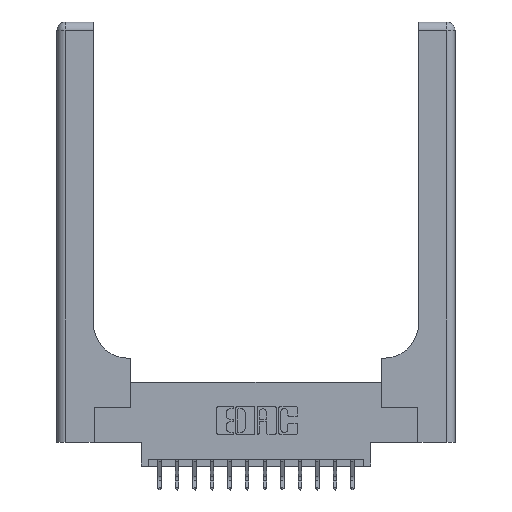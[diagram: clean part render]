
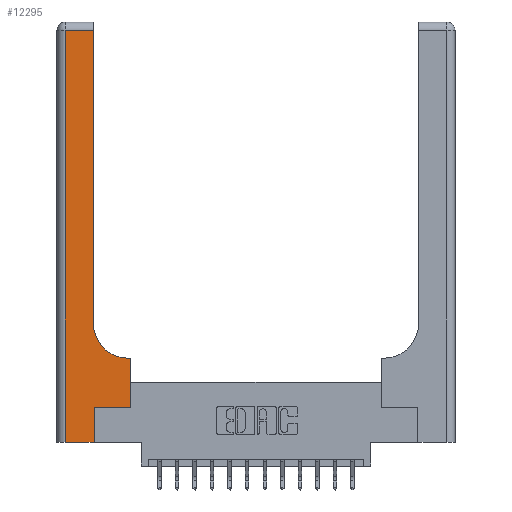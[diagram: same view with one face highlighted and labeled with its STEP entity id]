
A CAD part, top view. The second image highlights one B-rep face of the part: STEP entity #12295.
In plain terms, the highlighted planar face has unit normal (0, 0, 1).
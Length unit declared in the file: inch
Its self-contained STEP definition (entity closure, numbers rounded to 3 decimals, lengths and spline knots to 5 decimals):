
#17 = VECTOR ( 'NONE', #10789, 39.37008 ) ;
#334 = LINE ( 'NONE', #4444, #10123 ) ;
#576 = LINE ( 'NONE', #14651, #10993 ) ;
#1118 = VERTEX_POINT ( 'NONE', #5694 ) ;
#1309 = AXIS2_PLACEMENT_3D ( 'NONE', #10838, #9506, #16489 ) ;
#1325 = VERTEX_POINT ( 'NONE', #16546 ) ;
#1569 = ORIENTED_EDGE ( 'NONE', *, *, #14735, .T. ) ;
#2502 = VERTEX_POINT ( 'NONE', #8086 ) ;
#2768 = EDGE_CURVE ( 'NONE', #1325, #4122, #14981, .T. ) ;
#3259 = DIRECTION ( 'NONE',  ( 0., -1., 0. ) ) ;
#3391 = LINE ( 'NONE', #16825, #10990 ) ;
#3487 = AXIS2_PLACEMENT_3D ( 'NONE', #13956, #15382, #6989 ) ;
#3611 = CARTESIAN_POINT ( 'NONE',  ( 0.06, 0., 0.37 ) ) ;
#3619 = LINE ( 'NONE', #14592, #6126 ) ;
#3621 = ORIENTED_EDGE ( 'NONE', *, *, #2768, .T. ) ;
#4122 = VERTEX_POINT ( 'NONE', #6621 ) ;
#4444 = CARTESIAN_POINT ( 'NONE',  ( 0.06, 3., 0.37 ) ) ;
#4776 = ORIENTED_EDGE ( 'NONE', *, *, #13114, .T. ) ;
#4876 = EDGE_CURVE ( 'NONE', #17245, #13793, #6513, .T. ) ;
#4936 = EDGE_CURVE ( 'NONE', #9885, #12798, #14653, .T. ) ;
#5588 = CARTESIAN_POINT ( 'NONE',  ( 0.528, 0.25, 0.37 ) ) ;
#5694 = CARTESIAN_POINT ( 'NONE',  ( 0.06, 2.94, 0.37 ) ) ;
#5962 = DIRECTION ( 'NONE',  ( 1., 0., 0. ) ) ;
#6100 = VECTOR ( 'NONE', #9036, 39.37008 ) ;
#6126 = VECTOR ( 'NONE', #8880, 39.37008 ) ;
#6250 = DIRECTION ( 'NONE',  ( -1., 0., 0. ) ) ;
#6513 = LINE ( 'NONE', #10456, #6100 ) ;
#6621 = CARTESIAN_POINT ( 'NONE',  ( 0.26, 2.94, 0.37 ) ) ;
#6989 = DIRECTION ( 'NONE',  ( -1., 0., 0. ) ) ;
#7550 = VECTOR ( 'NONE', #14741, 39.37008 ) ;
#7786 = EDGE_CURVE ( 'NONE', #2502, #17245, #3391, .T. ) ;
#8086 = CARTESIAN_POINT ( 'NONE',  ( 0.265, 0.25, 0.37 ) ) ;
#8865 = CIRCLE ( 'NONE', #1309, 0.25 ) ;
#8880 = DIRECTION ( 'NONE',  ( -1., 0., 0. ) ) ;
#9036 = DIRECTION ( 'NONE',  ( 0., 1., 0. ) ) ;
#9077 = CARTESIAN_POINT ( 'NONE',  ( 0.265, 0., 0.37 ) ) ;
#9306 = CARTESIAN_POINT ( 'NONE',  ( 0., 0., 0.37 ) ) ;
#9506 = DIRECTION ( 'NONE',  ( 0., 0., -1. ) ) ;
#9885 = VERTEX_POINT ( 'NONE', #3611 ) ;
#10052 = EDGE_CURVE ( 'NONE', #14699, #1325, #8865, .T. ) ;
#10123 = VECTOR ( 'NONE', #3259, 39.37008 ) ;
#10176 = ORIENTED_EDGE ( 'NONE', *, *, #4876, .T. ) ;
#10443 = ORIENTED_EDGE ( 'NONE', *, *, #16587, .T. ) ;
#10456 = CARTESIAN_POINT ( 'NONE',  ( 0.528, 0.25, 0.37 ) ) ;
#10625 = CARTESIAN_POINT ( 'NONE',  ( 0.51, 0.6, 0.37 ) ) ;
#10789 = DIRECTION ( 'NONE',  ( 0., 1., 0. ) ) ;
#10838 = CARTESIAN_POINT ( 'NONE',  ( 0.51, 0.85, 0.37 ) ) ;
#10990 = VECTOR ( 'NONE', #5962, 39.37008 ) ;
#10993 = VECTOR ( 'NONE', #14485, 39.37008 ) ;
#12072 = CARTESIAN_POINT ( 'NONE',  ( 0.528, 0.6, 0.37 ) ) ;
#12295 = ADVANCED_FACE ( 'NONE', ( #16493 ), #12616, .F. ) ;
#12616 = PLANE ( 'NONE',  #3487 ) ;
#12798 = VERTEX_POINT ( 'NONE', #9077 ) ;
#13114 = EDGE_CURVE ( 'NONE', #13793, #14699, #3619, .T. ) ;
#13464 = CARTESIAN_POINT ( 'NONE',  ( 0.26, 3., 0.37 ) ) ;
#13793 = VERTEX_POINT ( 'NONE', #12072 ) ;
#13956 = CARTESIAN_POINT ( 'NONE',  ( 0., 3., 0.37 ) ) ;
#14485 = DIRECTION ( 'NONE',  ( 0., 1., 0. ) ) ;
#14575 = EDGE_CURVE ( 'NONE', #12798, #2502, #576, .T. ) ;
#14592 = CARTESIAN_POINT ( 'NONE',  ( 0.26, 0.6, 0.37 ) ) ;
#14651 = CARTESIAN_POINT ( 'NONE',  ( 0.265, 0., 0.37 ) ) ;
#14653 = LINE ( 'NONE', #9306, #7550 ) ;
#14699 = VERTEX_POINT ( 'NONE', #10625 ) ;
#14735 = EDGE_CURVE ( 'NONE', #1118, #9885, #334, .T. ) ;
#14741 = DIRECTION ( 'NONE',  ( 1., 0., 0. ) ) ;
#14948 = ORIENTED_EDGE ( 'NONE', *, *, #14575, .T. ) ;
#14981 = LINE ( 'NONE', #13464, #17 ) ;
#15382 = DIRECTION ( 'NONE',  ( 0., 0., -1. ) ) ;
#16022 = CARTESIAN_POINT ( 'NONE',  ( 0., 2.94, 0.37 ) ) ;
#16350 = ORIENTED_EDGE ( 'NONE', *, *, #4936, .T. ) ;
#16484 = ORIENTED_EDGE ( 'NONE', *, *, #10052, .T. ) ;
#16489 = DIRECTION ( 'NONE',  ( 1., 0., 0. ) ) ;
#16493 = FACE_OUTER_BOUND ( 'NONE', #17357, .T. ) ;
#16546 = CARTESIAN_POINT ( 'NONE',  ( 0.26, 0.85, 0.37 ) ) ;
#16587 = EDGE_CURVE ( 'NONE', #4122, #1118, #17102, .T. ) ;
#16825 = CARTESIAN_POINT ( 'NONE',  ( 0.265, 0.25, 0.37 ) ) ;
#17102 = LINE ( 'NONE', #16022, #17645 ) ;
#17245 = VERTEX_POINT ( 'NONE', #5588 ) ;
#17311 = ORIENTED_EDGE ( 'NONE', *, *, #7786, .T. ) ;
#17357 = EDGE_LOOP ( 'NONE', ( #3621, #10443, #1569, #16350, #14948, #17311, #10176, #4776, #16484 ) ) ;
#17645 = VECTOR ( 'NONE', #6250, 39.37008 ) ;
